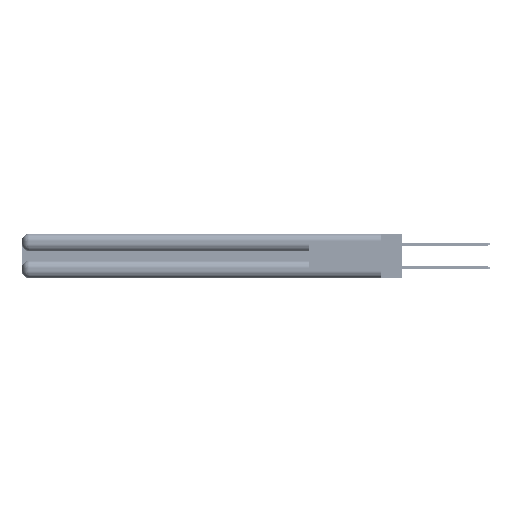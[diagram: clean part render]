
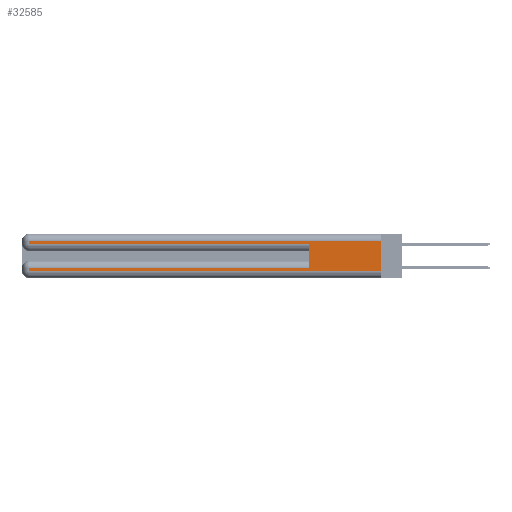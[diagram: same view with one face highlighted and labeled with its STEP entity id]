
A CAD part, left-side view. The second image highlights one B-rep face of the part: STEP entity #32585.
In plain terms, the highlighted planar face has unit normal (-1, 0, 0).
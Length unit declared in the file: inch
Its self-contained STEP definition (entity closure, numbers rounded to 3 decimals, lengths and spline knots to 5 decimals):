
#1534 = CARTESIAN_POINT ( 'NONE',  ( 0., 2.94, 0.31 ) ) ;
#3614 = VERTEX_POINT ( 'NONE', #37139 ) ;
#4224 = EDGE_CURVE ( 'NONE', #27952, #23744, #40102, .T. ) ;
#4227 = CARTESIAN_POINT ( 'NONE',  ( 0., 0., 0.37 ) ) ;
#4451 = ORIENTED_EDGE ( 'NONE', *, *, #38718, .T. ) ;
#4931 = ORIENTED_EDGE ( 'NONE', *, *, #41202, .T. ) ;
#5340 = VECTOR ( 'NONE', #8074, 39.37008 ) ;
#5631 = EDGE_CURVE ( 'NONE', #27476, #21020, #18687, .T. ) ;
#6017 = VECTOR ( 'NONE', #54547, 39.37008 ) ;
#6389 = CARTESIAN_POINT ( 'NONE',  ( 0., 0., 0.085 ) ) ;
#6910 = FACE_OUTER_BOUND ( 'NONE', #54895, .T. ) ;
#7236 = VECTOR ( 'NONE', #29905, 39.37008 ) ;
#8074 = DIRECTION ( 'NONE',  ( 0., 0., 1. ) ) ;
#9244 = CARTESIAN_POINT ( 'NONE',  ( 0., 0., 0.285 ) ) ;
#9531 = VECTOR ( 'NONE', #37796, 39.37008 ) ;
#13054 = VECTOR ( 'NONE', #47847, 39.37008 ) ;
#13748 = VERTEX_POINT ( 'NONE', #1534 ) ;
#14236 = CARTESIAN_POINT ( 'NONE',  ( 0., 0., 0.31 ) ) ;
#18539 = DIRECTION ( 'NONE',  ( 0., 1., 0. ) ) ;
#18687 = LINE ( 'NONE', #4227, #7236 ) ;
#20403 = DIRECTION ( 'NONE',  ( 0., 0., -1. ) ) ;
#20705 = LINE ( 'NONE', #9244, #41930 ) ;
#21020 = VERTEX_POINT ( 'NONE', #29065 ) ;
#21147 = VECTOR ( 'NONE', #18539, 39.37008 ) ;
#23610 = EDGE_CURVE ( 'NONE', #13748, #40717, #24422, .T. ) ;
#23744 = VERTEX_POINT ( 'NONE', #40432 ) ;
#24422 = LINE ( 'NONE', #30660, #13054 ) ;
#24926 = AXIS2_PLACEMENT_3D ( 'NONE', #28745, #45780, #20403 ) ;
#25036 = CARTESIAN_POINT ( 'NONE',  ( 0., 2.94, 0.37 ) ) ;
#25505 = ORIENTED_EDGE ( 'NONE', *, *, #4224, .T. ) ;
#26683 = VECTOR ( 'NONE', #36288, 39.37008 ) ;
#26833 = LINE ( 'NONE', #29379, #5340 ) ;
#27476 = VERTEX_POINT ( 'NONE', #44267 ) ;
#27952 = VERTEX_POINT ( 'NONE', #31252 ) ;
#28745 = CARTESIAN_POINT ( 'NONE',  ( 0., 0., 0.37 ) ) ;
#29065 = CARTESIAN_POINT ( 'NONE',  ( 0., 0., 0.06 ) ) ;
#29379 = CARTESIAN_POINT ( 'NONE',  ( 0., 0.6, 0.145 ) ) ;
#29681 = CARTESIAN_POINT ( 'NONE',  ( 0., 0.6, 0.285 ) ) ;
#29905 = DIRECTION ( 'NONE',  ( 0., 0., -1. ) ) ;
#30600 = CARTESIAN_POINT ( 'NONE',  ( 0., 2.94, 0.285 ) ) ;
#30660 = CARTESIAN_POINT ( 'NONE',  ( 0., 2.94, 0.37 ) ) ;
#31252 = CARTESIAN_POINT ( 'NONE',  ( 0., 2.94, 0.085 ) ) ;
#32585 = ADVANCED_FACE ( 'NONE', ( #6910 ), #37287, .F. ) ;
#33681 = ORIENTED_EDGE ( 'NONE', *, *, #5631, .F. ) ;
#35341 = ORIENTED_EDGE ( 'NONE', *, *, #49105, .T. ) ;
#35747 = ORIENTED_EDGE ( 'NONE', *, *, #23610, .T. ) ;
#36288 = DIRECTION ( 'NONE',  ( 0., 1., 0. ) ) ;
#37139 = CARTESIAN_POINT ( 'NONE',  ( 0., 0.6, 0.085 ) ) ;
#37287 = PLANE ( 'NONE',  #24926 ) ;
#37796 = DIRECTION ( 'NONE',  ( 0., -1., 0. ) ) ;
#38718 = EDGE_CURVE ( 'NONE', #27476, #13748, #54834, .T. ) ;
#40102 = LINE ( 'NONE', #25036, #6017 ) ;
#40432 = CARTESIAN_POINT ( 'NONE',  ( 0., 2.94, 0.06 ) ) ;
#40717 = VERTEX_POINT ( 'NONE', #30600 ) ;
#41202 = EDGE_CURVE ( 'NONE', #23744, #21020, #42221, .T. ) ;
#41930 = VECTOR ( 'NONE', #47569, 39.37008 ) ;
#42221 = LINE ( 'NONE', #50296, #9531 ) ;
#44267 = CARTESIAN_POINT ( 'NONE',  ( 0., 0., 0.31 ) ) ;
#44544 = VERTEX_POINT ( 'NONE', #29681 ) ;
#45780 = DIRECTION ( 'NONE',  ( 1., 0., 0. ) ) ;
#47569 = DIRECTION ( 'NONE',  ( 0., -1., 0. ) ) ;
#47607 = EDGE_CURVE ( 'NONE', #3614, #44544, #26833, .T. ) ;
#47702 = ORIENTED_EDGE ( 'NONE', *, *, #47607, .F. ) ;
#47847 = DIRECTION ( 'NONE',  ( 0., 0., -1. ) ) ;
#48878 = EDGE_CURVE ( 'NONE', #40717, #44544, #20705, .T. ) ;
#49105 = EDGE_CURVE ( 'NONE', #3614, #27952, #55049, .T. ) ;
#50296 = CARTESIAN_POINT ( 'NONE',  ( 0., 0., 0.06 ) ) ;
#53625 = ORIENTED_EDGE ( 'NONE', *, *, #48878, .T. ) ;
#54547 = DIRECTION ( 'NONE',  ( 0., 0., -1. ) ) ;
#54834 = LINE ( 'NONE', #14236, #21147 ) ;
#54895 = EDGE_LOOP ( 'NONE', ( #33681, #4451, #35747, #53625, #47702, #35341, #25505, #4931 ) ) ;
#55049 = LINE ( 'NONE', #6389, #26683 ) ;
